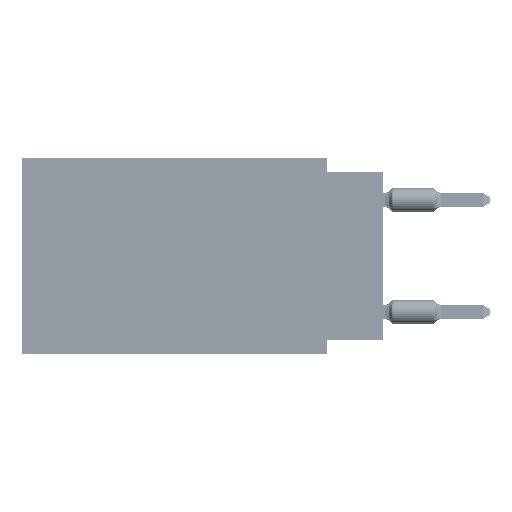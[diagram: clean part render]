
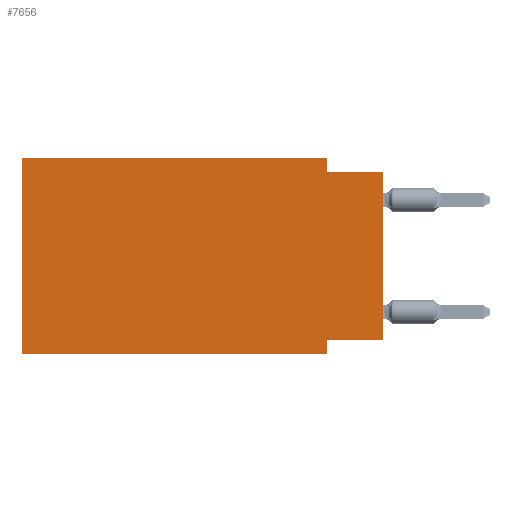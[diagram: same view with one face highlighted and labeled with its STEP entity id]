
A CAD part, left-side view. The second image highlights one B-rep face of the part: STEP entity #7656.
In plain terms, the highlighted planar face has unit normal (-1, 0, 0).
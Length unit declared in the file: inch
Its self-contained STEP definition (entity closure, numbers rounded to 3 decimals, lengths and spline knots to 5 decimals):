
#2117 = DIRECTION ( 'NONE',  ( 0., 0., -1. ) ) ;
#4369 = EDGE_CURVE ( 'NONE', #56196, #7206, #25686, .T. ) ;
#4520 = CARTESIAN_POINT ( 'NONE',  ( 0., 0.1, -0.025 ) ) ;
#5992 = CARTESIAN_POINT ( 'NONE',  ( 0., 0., -0.025 ) ) ;
#6324 = VERTEX_POINT ( 'NONE', #21300 ) ;
#7206 = VERTEX_POINT ( 'NONE', #5992 ) ;
#7326 = DIRECTION ( 'NONE',  ( 0., 0., 1. ) ) ;
#7656 = ADVANCED_FACE ( 'NONE', ( #58252 ), #12394, .F. ) ;
#7786 = ORIENTED_EDGE ( 'NONE', *, *, #25172, .F. ) ;
#10215 = VECTOR ( 'NONE', #36515, 39.37008 ) ;
#10774 = EDGE_CURVE ( 'NONE', #49425, #59371, #47110, .T. ) ;
#12394 = PLANE ( 'NONE',  #33943 ) ;
#13127 = CARTESIAN_POINT ( 'NONE',  ( 0., 0., 0. ) ) ;
#13378 = CARTESIAN_POINT ( 'NONE',  ( 0., 0., -0.325 ) ) ;
#13964 = ORIENTED_EDGE ( 'NONE', *, *, #55078, .T. ) ;
#15530 = LINE ( 'NONE', #47299, #22541 ) ;
#16838 = CARTESIAN_POINT ( 'NONE',  ( 0., 0.1, -0.325 ) ) ;
#16915 = VECTOR ( 'NONE', #7326, 39.37008 ) ;
#17960 = ORIENTED_EDGE ( 'NONE', *, *, #45837, .T. ) ;
#20416 = ORIENTED_EDGE ( 'NONE', *, *, #37118, .F. ) ;
#21300 = CARTESIAN_POINT ( 'NONE',  ( 0., 0.645, 0. ) ) ;
#21655 = DIRECTION ( 'NONE',  ( 0., -1., 0. ) ) ;
#22541 = VECTOR ( 'NONE', #21655, 39.37008 ) ;
#23072 = LINE ( 'NONE', #13127, #16915 ) ;
#25172 = EDGE_CURVE ( 'NONE', #42154, #49425, #53856, .T. ) ;
#25686 = LINE ( 'NONE', #46540, #57777 ) ;
#25813 = VECTOR ( 'NONE', #52110, 39.37008 ) ;
#28311 = EDGE_CURVE ( 'NONE', #6324, #35415, #41484, .T. ) ;
#29636 = CARTESIAN_POINT ( 'NONE',  ( 0., 0.1, -0.35 ) ) ;
#31230 = CARTESIAN_POINT ( 'NONE',  ( 0., 0.645, 0. ) ) ;
#33943 = AXIS2_PLACEMENT_3D ( 'NONE', #44205, #65095, #2117 ) ;
#35415 = VERTEX_POINT ( 'NONE', #60896 ) ;
#36515 = DIRECTION ( 'NONE',  ( 0., 0., -1. ) ) ;
#37118 = EDGE_CURVE ( 'NONE', #35415, #56196, #53233, .T. ) ;
#37585 = EDGE_CURVE ( 'NONE', #50374, #6324, #47655, .T. ) ;
#37738 = DIRECTION ( 'NONE',  ( 0., 0., 1. ) ) ;
#41408 = DIRECTION ( 'NONE',  ( 0., -1., 0. ) ) ;
#41484 = LINE ( 'NONE', #31230, #25813 ) ;
#42154 = VERTEX_POINT ( 'NONE', #62876 ) ;
#42645 = CARTESIAN_POINT ( 'NONE',  ( 0., 0.1, -0.35 ) ) ;
#43039 = VECTOR ( 'NONE', #59706, 39.37008 ) ;
#44099 = EDGE_LOOP ( 'NONE', ( #17960, #48081, #20416, #65937, #57493, #13964, #48750, #7786 ) ) ;
#44205 = CARTESIAN_POINT ( 'NONE',  ( 0., 0.645, 0. ) ) ;
#45837 = EDGE_CURVE ( 'NONE', #42154, #7206, #23072, .T. ) ;
#46540 = CARTESIAN_POINT ( 'NONE',  ( 0., 0., -0.025 ) ) ;
#47110 = LINE ( 'NONE', #42645, #10215 ) ;
#47299 = CARTESIAN_POINT ( 'NONE',  ( 0., 0.645, -0.35 ) ) ;
#47655 = LINE ( 'NONE', #64085, #60554 ) ;
#48081 = ORIENTED_EDGE ( 'NONE', *, *, #4369, .F. ) ;
#48750 = ORIENTED_EDGE ( 'NONE', *, *, #10774, .F. ) ;
#49425 = VERTEX_POINT ( 'NONE', #16838 ) ;
#50374 = VERTEX_POINT ( 'NONE', #65892 ) ;
#52110 = DIRECTION ( 'NONE',  ( 0., -1., 0. ) ) ;
#53233 = LINE ( 'NONE', #59017, #43039 ) ;
#53856 = LINE ( 'NONE', #13378, #55060 ) ;
#55060 = VECTOR ( 'NONE', #57969, 39.37008 ) ;
#55078 = EDGE_CURVE ( 'NONE', #50374, #59371, #15530, .T. ) ;
#56196 = VERTEX_POINT ( 'NONE', #4520 ) ;
#57493 = ORIENTED_EDGE ( 'NONE', *, *, #37585, .F. ) ;
#57777 = VECTOR ( 'NONE', #41408, 39.37008 ) ;
#57969 = DIRECTION ( 'NONE',  ( 0., 1., 0. ) ) ;
#58252 = FACE_OUTER_BOUND ( 'NONE', #44099, .T. ) ;
#59017 = CARTESIAN_POINT ( 'NONE',  ( 0., 0.1, 0. ) ) ;
#59371 = VERTEX_POINT ( 'NONE', #29636 ) ;
#59706 = DIRECTION ( 'NONE',  ( 0., 0., -1. ) ) ;
#60554 = VECTOR ( 'NONE', #37738, 39.37008 ) ;
#60896 = CARTESIAN_POINT ( 'NONE',  ( 0., 0.1, 0. ) ) ;
#62876 = CARTESIAN_POINT ( 'NONE',  ( 0., 0., -0.325 ) ) ;
#64085 = CARTESIAN_POINT ( 'NONE',  ( 0., 0.645, 0. ) ) ;
#65095 = DIRECTION ( 'NONE',  ( 1., 0., 0. ) ) ;
#65892 = CARTESIAN_POINT ( 'NONE',  ( 0., 0.645, -0.35 ) ) ;
#65937 = ORIENTED_EDGE ( 'NONE', *, *, #28311, .F. ) ;
